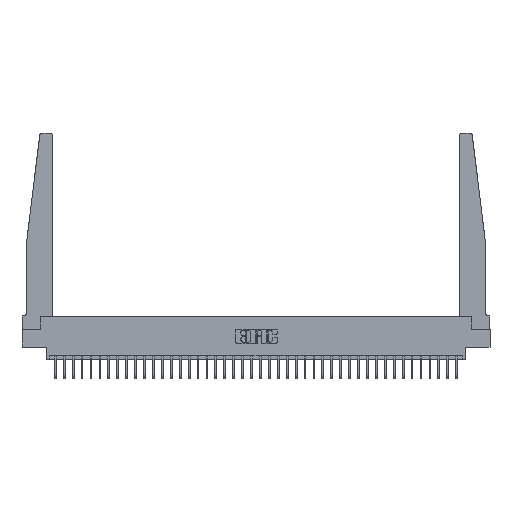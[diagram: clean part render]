
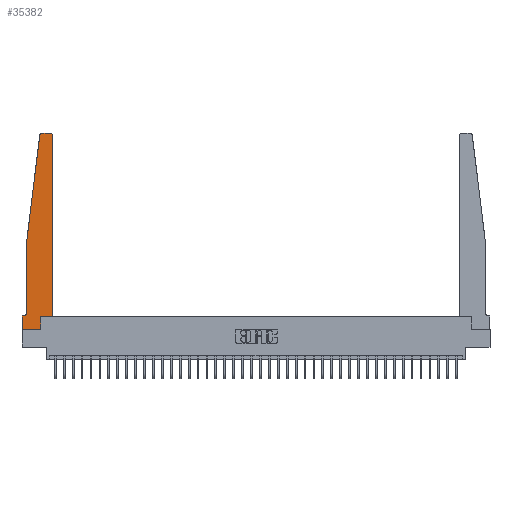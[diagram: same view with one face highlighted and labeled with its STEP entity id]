
A CAD part, top view. The second image highlights one B-rep face of the part: STEP entity #35382.
In plain terms, the highlighted planar face has unit normal (0, 0, 1).
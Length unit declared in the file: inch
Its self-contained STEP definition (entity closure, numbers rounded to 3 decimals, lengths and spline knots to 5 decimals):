
#146 = CARTESIAN_POINT ( 'NONE',  ( 0., 0., 0.37 ) ) ;
#1398 = LINE ( 'NONE', #11478, #12291 ) ;
#2427 = EDGE_CURVE ( 'NONE', #30847, #32865, #5102, .T. ) ;
#3252 = DIRECTION ( 'NONE',  ( -1., 0., 0. ) ) ;
#3516 = VECTOR ( 'NONE', #16792, 39.37008 ) ;
#4171 = CARTESIAN_POINT ( 'NONE',  ( 0., 0.1875, 0.37 ) ) ;
#4292 = PLANE ( 'NONE',  #11399 ) ;
#4407 = ORIENTED_EDGE ( 'NONE', *, *, #5156, .T. ) ;
#4921 = CARTESIAN_POINT ( 'NONE',  ( 0.425, 0.18, 0.37 ) ) ;
#4928 = EDGE_LOOP ( 'NONE', ( #4407, #25430, #17969, #10567, #22004, #12152, #15782, #19605, #33840, #33680, #14539, #17489 ) ) ;
#5102 = LINE ( 'NONE', #22775, #17211 ) ;
#5148 = CARTESIAN_POINT ( 'NONE',  ( 0.2605, 0., 0.37 ) ) ;
#5156 = EDGE_CURVE ( 'NONE', #6254, #29346, #1398, .T. ) ;
#5837 = VERTEX_POINT ( 'NONE', #23191 ) ;
#6199 = EDGE_CURVE ( 'NONE', #18394, #18873, #30148, .T. ) ;
#6254 = VERTEX_POINT ( 'NONE', #11003 ) ;
#7140 = DIRECTION ( 'NONE',  ( 1., 0., 0. ) ) ;
#7614 = DIRECTION ( 'NONE',  ( 0., 0., 1. ) ) ;
#7747 = CARTESIAN_POINT ( 'NONE',  ( 0.425, 2.72, 0.37 ) ) ;
#8130 = DIRECTION ( 'NONE',  ( 0., -1., 0. ) ) ;
#8569 = LINE ( 'NONE', #4921, #23377 ) ;
#8634 = DIRECTION ( 'NONE',  ( -1., 0., 0. ) ) ;
#8824 = LINE ( 'NONE', #17547, #31102 ) ;
#9215 = AXIS2_PLACEMENT_3D ( 'NONE', #35148, #7614, #29821 ) ;
#9342 = EDGE_CURVE ( 'NONE', #12669, #18394, #14367, .T. ) ;
#9916 = CARTESIAN_POINT ( 'NONE',  ( 0.065, 1.25, 0.37 ) ) ;
#10375 = VERTEX_POINT ( 'NONE', #26101 ) ;
#10567 = ORIENTED_EDGE ( 'NONE', *, *, #28658, .T. ) ;
#10734 = CARTESIAN_POINT ( 'NONE',  ( 0.425, 0.18, 0.37 ) ) ;
#11003 = CARTESIAN_POINT ( 'NONE',  ( 0.395, 2.75, 0.37 ) ) ;
#11042 = EDGE_CURVE ( 'NONE', #29346, #33778, #14229, .T. ) ;
#11399 = AXIS2_PLACEMENT_3D ( 'NONE', #4171, #15208, #12299 ) ;
#11478 = CARTESIAN_POINT ( 'NONE',  ( 0.25, 2.75, 0.37 ) ) ;
#12152 = ORIENTED_EDGE ( 'NONE', *, *, #9342, .T. ) ;
#12153 = EDGE_CURVE ( 'NONE', #32865, #10375, #8569, .T. ) ;
#12291 = VECTOR ( 'NONE', #20183, 39.37008 ) ;
#12299 = DIRECTION ( 'NONE',  ( 1., 0., 0. ) ) ;
#12669 = VERTEX_POINT ( 'NONE', #34245 ) ;
#13768 = FACE_OUTER_BOUND ( 'NONE', #4928, .T. ) ;
#14186 = CARTESIAN_POINT ( 'NONE',  ( 0.065, 0.1875, 0.37 ) ) ;
#14229 = CIRCLE ( 'NONE', #30858, 0.03 ) ;
#14367 = LINE ( 'NONE', #14186, #34096 ) ;
#14539 = ORIENTED_EDGE ( 'NONE', *, *, #28083, .T. ) ;
#14711 = VECTOR ( 'NONE', #8130, 39.37008 ) ;
#15208 = DIRECTION ( 'NONE',  ( 0., 0., 1. ) ) ;
#15782 = ORIENTED_EDGE ( 'NONE', *, *, #6199, .T. ) ;
#16792 = DIRECTION ( 'NONE',  ( 0., -1., 0. ) ) ;
#16803 = CARTESIAN_POINT ( 'NONE',  ( 0.24675, 2.72367, 0.37 ) ) ;
#17201 = EDGE_CURVE ( 'NONE', #17249, #6254, #26001, .T. ) ;
#17211 = VECTOR ( 'NONE', #31239, 39.37008 ) ;
#17249 = VERTEX_POINT ( 'NONE', #7747 ) ;
#17489 = ORIENTED_EDGE ( 'NONE', *, *, #17201, .T. ) ;
#17547 = CARTESIAN_POINT ( 'NONE',  ( 0., 0., 0.37 ) ) ;
#17744 = LINE ( 'NONE', #19073, #14711 ) ;
#17969 = ORIENTED_EDGE ( 'NONE', *, *, #20819, .T. ) ;
#18394 = VERTEX_POINT ( 'NONE', #22942 ) ;
#18873 = VERTEX_POINT ( 'NONE', #22590 ) ;
#19073 = CARTESIAN_POINT ( 'NONE',  ( 0.065, 1.25, 0.37 ) ) ;
#19605 = ORIENTED_EDGE ( 'NONE', *, *, #20605, .T. ) ;
#19623 = LINE ( 'NONE', #10734, #27942 ) ;
#20183 = DIRECTION ( 'NONE',  ( -1., 0., 0. ) ) ;
#20605 = EDGE_CURVE ( 'NONE', #18873, #30847, #8824, .T. ) ;
#20819 = EDGE_CURVE ( 'NONE', #33778, #5837, #28449, .T. ) ;
#20997 = VECTOR ( 'NONE', #24243, 39.37008 ) ;
#22004 = ORIENTED_EDGE ( 'NONE', *, *, #31056, .T. ) ;
#22590 = CARTESIAN_POINT ( 'NONE',  ( 0., 0., 0.37 ) ) ;
#22775 = CARTESIAN_POINT ( 'NONE',  ( 0.2605, 0.18, 0.37 ) ) ;
#22942 = CARTESIAN_POINT ( 'NONE',  ( 0., 0.1875, 0.37 ) ) ;
#23191 = CARTESIAN_POINT ( 'NONE',  ( 0.065, 1.25, 0.37 ) ) ;
#23377 = VECTOR ( 'NONE', #30146, 39.37008 ) ;
#24124 = CIRCLE ( 'NONE', #25309, 0.05 ) ;
#24243 = DIRECTION ( 'NONE',  ( -0.122, -0.992, 0. ) ) ;
#25309 = AXIS2_PLACEMENT_3D ( 'NONE', #25785, #31335, #8634 ) ;
#25430 = ORIENTED_EDGE ( 'NONE', *, *, #11042, .T. ) ;
#25767 = CARTESIAN_POINT ( 'NONE',  ( 0.27653, 2.72, 0.37 ) ) ;
#25785 = CARTESIAN_POINT ( 'NONE',  ( 0.015, 0.2375, 0.37 ) ) ;
#26001 = CIRCLE ( 'NONE', #9215, 0.03 ) ;
#26101 = CARTESIAN_POINT ( 'NONE',  ( 0.425, 0.18, 0.37 ) ) ;
#26389 = CARTESIAN_POINT ( 'NONE',  ( 0.27653, 2.75, 0.37 ) ) ;
#27569 = DIRECTION ( 'NONE',  ( 0., 1., 0. ) ) ;
#27942 = VECTOR ( 'NONE', #27569, 39.37008 ) ;
#28083 = EDGE_CURVE ( 'NONE', #10375, #17249, #19623, .T. ) ;
#28449 = LINE ( 'NONE', #9916, #20997 ) ;
#28610 = DIRECTION ( 'NONE',  ( 1., 0., 0. ) ) ;
#28658 = EDGE_CURVE ( 'NONE', #5837, #35138, #17744, .T. ) ;
#29346 = VERTEX_POINT ( 'NONE', #26389 ) ;
#29821 = DIRECTION ( 'NONE',  ( 1., 0., 0. ) ) ;
#29853 = CARTESIAN_POINT ( 'NONE',  ( 0.2605, 0.18, 0.37 ) ) ;
#30146 = DIRECTION ( 'NONE',  ( 1., 0., 0. ) ) ;
#30148 = LINE ( 'NONE', #146, #3516 ) ;
#30847 = VERTEX_POINT ( 'NONE', #5148 ) ;
#30858 = AXIS2_PLACEMENT_3D ( 'NONE', #25767, #31071, #28610 ) ;
#31056 = EDGE_CURVE ( 'NONE', #35138, #12669, #24124, .T. ) ;
#31071 = DIRECTION ( 'NONE',  ( 0., 0., 1. ) ) ;
#31102 = VECTOR ( 'NONE', #7140, 39.37008 ) ;
#31239 = DIRECTION ( 'NONE',  ( 0., 1., 0. ) ) ;
#31335 = DIRECTION ( 'NONE',  ( 0., 0., -1. ) ) ;
#32865 = VERTEX_POINT ( 'NONE', #29853 ) ;
#33680 = ORIENTED_EDGE ( 'NONE', *, *, #12153, .T. ) ;
#33778 = VERTEX_POINT ( 'NONE', #16803 ) ;
#33840 = ORIENTED_EDGE ( 'NONE', *, *, #2427, .T. ) ;
#34096 = VECTOR ( 'NONE', #3252, 39.37008 ) ;
#34245 = CARTESIAN_POINT ( 'NONE',  ( 0.015, 0.1875, 0.37 ) ) ;
#35138 = VERTEX_POINT ( 'NONE', #35544 ) ;
#35148 = CARTESIAN_POINT ( 'NONE',  ( 0.395, 2.72, 0.37 ) ) ;
#35382 = ADVANCED_FACE ( 'NONE', ( #13768 ), #4292, .T. ) ;
#35544 = CARTESIAN_POINT ( 'NONE',  ( 0.065, 0.2375, 0.37 ) ) ;
